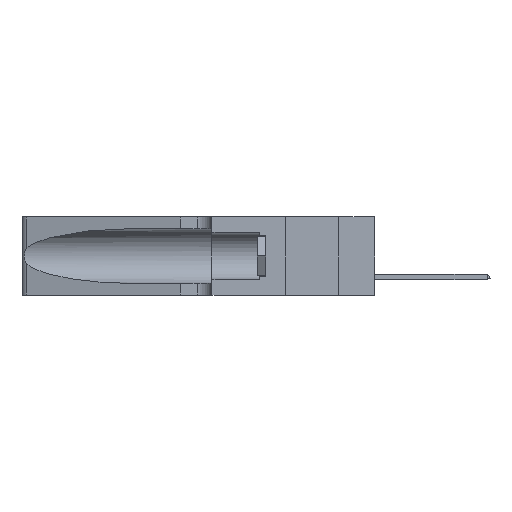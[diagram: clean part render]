
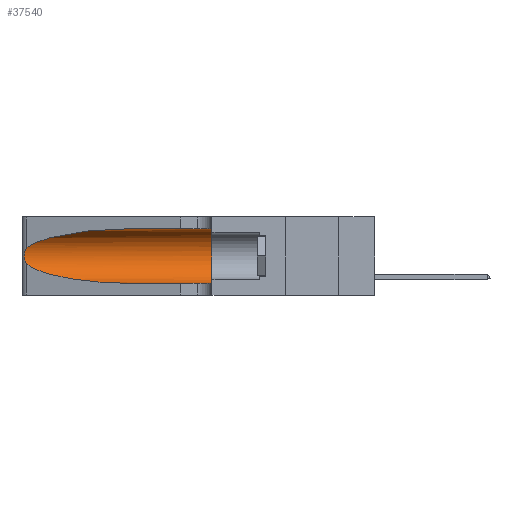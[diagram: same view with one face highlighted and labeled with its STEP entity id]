
A CAD part, left-side view. The second image highlights one B-rep face of the part: STEP entity #37540.
In plain terms, the highlighted cylindrical face has radius 3.308 mm (diameter 6.617 mm), a partial arc.
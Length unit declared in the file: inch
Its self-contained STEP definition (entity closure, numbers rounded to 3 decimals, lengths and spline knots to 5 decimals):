
#1360 = DIRECTION ( 'NONE',  ( 0., 1., 0. ) ) ;
#2076 = CARTESIAN_POINT ( 'NONE',  ( 0.26018, 1.23835, 0.19895 ) ) ;
#2791 = CARTESIAN_POINT ( 'NONE',  ( 0.25487, 1.22718, 0.14631 ) ) ;
#3043 = EDGE_CURVE ( 'NONE', #19501, #34234, #38832, .T. ) ;
#3107 = EDGE_CURVE ( 'NONE', #34234, #4500, #40358, .T. ) ;
#4500 = VERTEX_POINT ( 'NONE', #39067 ) ;
#5041 = AXIS2_PLACEMENT_3D ( 'NONE', #9771, #6190, #28914 ) ;
#5300 = CARTESIAN_POINT ( 'NONE',  ( 0.25487, 1.22718, 0.14631 ) ) ;
#6190 = DIRECTION ( 'NONE',  ( 0., -1., 0. ) ) ;
#6369 = VERTEX_POINT ( 'NONE', #17902 ) ;
#6499 = EDGE_LOOP ( 'NONE', ( #29747, #6510, #22245, #29742, #31012, #38569 ) ) ;
#6510 = ORIENTED_EDGE ( 'NONE', *, *, #37996, .T. ) ;
#6524 = CYLINDRICAL_SURFACE ( 'NONE', #5041, 0.13025 ) ;
#6613 =( BOUNDED_CURVE ( )  B_SPLINE_CURVE ( 3, ( #38966, #10637, #39814, #36614 ),
 .UNSPECIFIED., .F., .F. ) 
 B_SPLINE_CURVE_WITH_KNOTS ( ( 4, 4 ),
 ( 1.5708, 2.84003 ),
 .UNSPECIFIED. ) 
 CURVE ( )  GEOMETRIC_REPRESENTATION_ITEM ( )  RATIONAL_B_SPLINE_CURVE ( ( 1., 0.87, 0.87, 1. ) ) 
 REPRESENTATION_ITEM ( '' )  );
#7377 = CARTESIAN_POINT ( 'NONE',  ( 0.1305, 1.61858, 0.05475 ) ) ;
#8631 = CARTESIAN_POINT ( 'NONE',  ( 0.26017, 1.23833, 0.17102 ) ) ;
#8916 = CARTESIAN_POINT ( 'NONE',  ( 0.1305, 0.72297, 0.05475 ) ) ;
#9194 = CARTESIAN_POINT ( 'NONE',  ( 0.2373, 1.15595, 0.08982 ) ) ;
#9771 = CARTESIAN_POINT ( 'NONE',  ( 0.1305, 1.61858, 0.185 ) ) ;
#10637 = CARTESIAN_POINT ( 'NONE',  ( 0.18966, 0.96281, 0.31525 ) ) ;
#11116 = CARTESIAN_POINT ( 'NONE',  ( 0.1305, 1.61858, 0.31525 ) ) ;
#11422 = CARTESIAN_POINT ( 'NONE',  ( 0.25555, 1.22993, 0.14849 ) ) ;
#11704 = CARTESIAN_POINT ( 'NONE',  ( 0.25639, 1.23186, 0.15144 ) ) ;
#11826 = EDGE_CURVE ( 'NONE', #36977, #4500, #39715, .T. ) ;
#14081 = CARTESIAN_POINT ( 'NONE',  ( 0.1305, 0.35, 0.31525 ) ) ;
#14162 = AXIS2_PLACEMENT_3D ( 'NONE', #32898, #1360, #34877 ) ;
#14507 = CARTESIAN_POINT ( 'NONE',  ( 0.25787, 1.23484, 0.2124 ) ) ;
#14646 = CARTESIAN_POINT ( 'NONE',  ( 0.25487, 1.22718, 0.22369 ) ) ;
#14864 = VERTEX_POINT ( 'NONE', #20656 ) ;
#17902 = CARTESIAN_POINT ( 'NONE',  ( 0.1305, 0.72297, 0.31525 ) ) ;
#18966 = EDGE_CURVE ( 'NONE', #6369, #14864, #6613, .T. ) ;
#19501 = VERTEX_POINT ( 'NONE', #5300 ) ;
#20656 = CARTESIAN_POINT ( 'NONE',  ( 0.25487, 1.22718, 0.22369 ) ) ;
#20892 = VECTOR ( 'NONE', #29808, 39.37008 ) ;
#21370 = CARTESIAN_POINT ( 'NONE',  ( 0.25639, 1.23184, 0.21858 ) ) ;
#22245 = ORIENTED_EDGE ( 'NONE', *, *, #3043, .T. ) ;
#24178 = CARTESIAN_POINT ( 'NONE',  ( 0.26075, 1.23896, 0.178 ) ) ;
#24854 = CARTESIAN_POINT ( 'NONE',  ( 0.18966, 0.96281, 0.05475 ) ) ;
#24857 = CARTESIAN_POINT ( 'NONE',  ( 0.1305, 0.72297, 0.05475 ) ) ;
#27548 = FACE_OUTER_BOUND ( 'NONE', #6499, .T. ) ;
#27792 = CARTESIAN_POINT ( 'NONE',  ( 0.26075, 1.23896, 0.19203 ) ) ;
#28405 = B_SPLINE_CURVE_WITH_KNOTS ( 'NONE', 3,
 ( #14646, #36989, #21370, #14507, #30804, #2076, #27792, #24178, #8631, #40175, #30523, #11704, #11422, #30953 ),
 .UNSPECIFIED., .F., .F.,
 ( 4, 2, 2, 2, 2, 2, 4 ),
 ( 0., 0.00027, 0.00053, 0.00107, 0.0016, 0.00187, 0.00214 ),
 .UNSPECIFIED. ) ;
#28914 = DIRECTION ( 'NONE',  ( 0., 0., -1. ) ) ;
#29316 = VECTOR ( 'NONE', #33460, 39.37008 ) ;
#29742 = ORIENTED_EDGE ( 'NONE', *, *, #3107, .T. ) ;
#29747 = ORIENTED_EDGE ( 'NONE', *, *, #18966, .T. ) ;
#29808 = DIRECTION ( 'NONE',  ( 0., -1., 0. ) ) ;
#30523 = CARTESIAN_POINT ( 'NONE',  ( 0.25789, 1.23486, 0.15765 ) ) ;
#30804 = CARTESIAN_POINT ( 'NONE',  ( 0.25854, 1.2359, 0.20912 ) ) ;
#30953 = CARTESIAN_POINT ( 'NONE',  ( 0.25487, 1.22718, 0.14631 ) ) ;
#31012 = ORIENTED_EDGE ( 'NONE', *, *, #11826, .F. ) ;
#32898 = CARTESIAN_POINT ( 'NONE',  ( 0.1305, 0.35, 0.185 ) ) ;
#33460 = DIRECTION ( 'NONE',  ( 0., -1., 0. ) ) ;
#34234 = VERTEX_POINT ( 'NONE', #24857 ) ;
#34877 = DIRECTION ( 'NONE',  ( 0., 0., 1. ) ) ;
#35360 = LINE ( 'NONE', #11116, #20892 ) ;
#36614 = CARTESIAN_POINT ( 'NONE',  ( 0.25487, 1.22718, 0.22369 ) ) ;
#36977 = VERTEX_POINT ( 'NONE', #14081 ) ;
#36989 = CARTESIAN_POINT ( 'NONE',  ( 0.25555, 1.22994, 0.2215 ) ) ;
#37540 = ADVANCED_FACE ( 'NONE', ( #27548 ), #6524, .F. ) ;
#37996 = EDGE_CURVE ( 'NONE', #14864, #19501, #28405, .T. ) ;
#38569 = ORIENTED_EDGE ( 'NONE', *, *, #40435, .F. ) ;
#38832 =( BOUNDED_CURVE ( )  B_SPLINE_CURVE ( 3, ( #2791, #9194, #24854, #8916 ),
 .UNSPECIFIED., .F., .F. ) 
 B_SPLINE_CURVE_WITH_KNOTS ( ( 4, 4 ),
 ( 3.44316, 4.71239 ),
 .UNSPECIFIED. ) 
 CURVE ( )  GEOMETRIC_REPRESENTATION_ITEM ( )  RATIONAL_B_SPLINE_CURVE ( ( 1., 0.87, 0.87, 1. ) ) 
 REPRESENTATION_ITEM ( '' )  );
#38966 = CARTESIAN_POINT ( 'NONE',  ( 0.1305, 0.72297, 0.31525 ) ) ;
#39067 = CARTESIAN_POINT ( 'NONE',  ( 0.1305, 0.35, 0.05475 ) ) ;
#39715 = CIRCLE ( 'NONE', #14162, 0.13025 ) ;
#39814 = CARTESIAN_POINT ( 'NONE',  ( 0.2373, 1.15595, 0.28018 ) ) ;
#40175 = CARTESIAN_POINT ( 'NONE',  ( 0.25856, 1.23593, 0.16098 ) ) ;
#40358 = LINE ( 'NONE', #7377, #29316 ) ;
#40435 = EDGE_CURVE ( 'NONE', #6369, #36977, #35360, .T. ) ;
